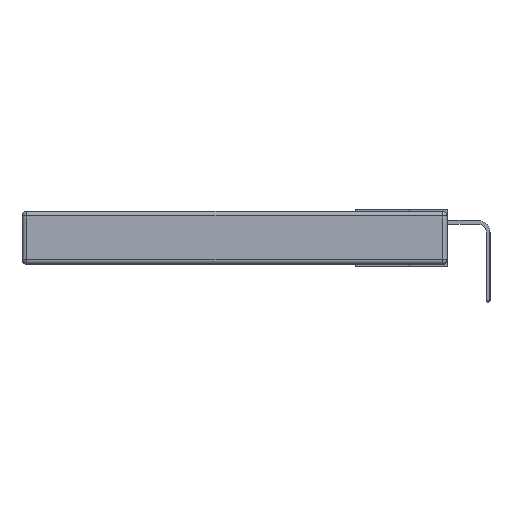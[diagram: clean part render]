
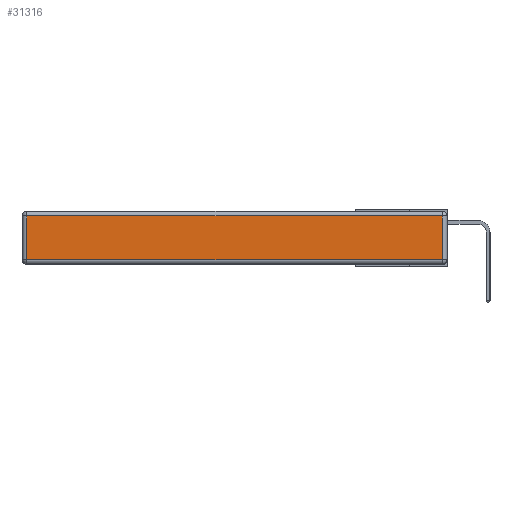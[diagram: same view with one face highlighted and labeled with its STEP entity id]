
A CAD part, left-side view. The second image highlights one B-rep face of the part: STEP entity #31316.
In plain terms, the highlighted planar face has unit normal (-1, 0, 0).
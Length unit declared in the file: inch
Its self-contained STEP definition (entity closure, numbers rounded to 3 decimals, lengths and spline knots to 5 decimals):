
#2116 = EDGE_LOOP ( 'NONE', ( #7819, #24639, #2526, #13981 ) ) ;
#2526 = ORIENTED_EDGE ( 'NONE', *, *, #8005, .T. ) ;
#2814 = DIRECTION ( 'NONE',  ( -1., 0., 0. ) ) ;
#3314 = EDGE_CURVE ( 'NONE', #15918, #26681, #12057, .T. ) ;
#7537 = DIRECTION ( 'NONE',  ( 0., 1., 0. ) ) ;
#7819 = ORIENTED_EDGE ( 'NONE', *, *, #3314, .T. ) ;
#8005 = EDGE_CURVE ( 'NONE', #9040, #12971, #25726, .T. ) ;
#9040 = VERTEX_POINT ( 'NONE', #17628 ) ;
#10610 = VECTOR ( 'NONE', #23692, 39.37008 ) ;
#12057 = LINE ( 'NONE', #32161, #32959 ) ;
#12971 = VERTEX_POINT ( 'NONE', #33990 ) ;
#13128 = LINE ( 'NONE', #17757, #10610 ) ;
#13981 = ORIENTED_EDGE ( 'NONE', *, *, #19170, .T. ) ;
#14454 = VECTOR ( 'NONE', #7537, 39.37008 ) ;
#15918 = VERTEX_POINT ( 'NONE', #27455 ) ;
#16862 = DIRECTION ( 'NONE',  ( 0., 0., -1. ) ) ;
#17628 = CARTESIAN_POINT ( 'NONE',  ( 0., 0.03, -0.03 ) ) ;
#17708 = FACE_OUTER_BOUND ( 'NONE', #2116, .T. ) ;
#17757 = CARTESIAN_POINT ( 'NONE',  ( 0., 0.03, -0.343 ) ) ;
#18188 = EDGE_CURVE ( 'NONE', #26681, #9040, #13128, .T. ) ;
#19170 = EDGE_CURVE ( 'NONE', #12971, #15918, #23115, .T. ) ;
#21216 = CARTESIAN_POINT ( 'NONE',  ( 0., 2.75, -0.03 ) ) ;
#21315 = DIRECTION ( 'NONE',  ( 0., 0., 1. ) ) ;
#21425 = PLANE ( 'NONE',  #30565 ) ;
#21529 = DIRECTION ( 'NONE',  ( 0., -1., 0. ) ) ;
#23115 = LINE ( 'NONE', #29812, #27663 ) ;
#23692 = DIRECTION ( 'NONE',  ( 0., 0., 1. ) ) ;
#24639 = ORIENTED_EDGE ( 'NONE', *, *, #18188, .T. ) ;
#25726 = LINE ( 'NONE', #21216, #14454 ) ;
#26681 = VERTEX_POINT ( 'NONE', #31909 ) ;
#27455 = CARTESIAN_POINT ( 'NONE',  ( 0., 2.72, -0.313 ) ) ;
#27663 = VECTOR ( 'NONE', #16862, 39.37008 ) ;
#29812 = CARTESIAN_POINT ( 'NONE',  ( 0., 2.72, -0.343 ) ) ;
#30565 = AXIS2_PLACEMENT_3D ( 'NONE', #32285, #2814, #21315 ) ;
#31316 = ADVANCED_FACE ( 'NONE', ( #17708 ), #21425, .T. ) ;
#31909 = CARTESIAN_POINT ( 'NONE',  ( 0., 0.03, -0.313 ) ) ;
#32161 = CARTESIAN_POINT ( 'NONE',  ( 0., 0., -0.313 ) ) ;
#32285 = CARTESIAN_POINT ( 'NONE',  ( 0., 0., -0.343 ) ) ;
#32959 = VECTOR ( 'NONE', #21529, 39.37008 ) ;
#33990 = CARTESIAN_POINT ( 'NONE',  ( 0., 2.72, -0.03 ) ) ;
